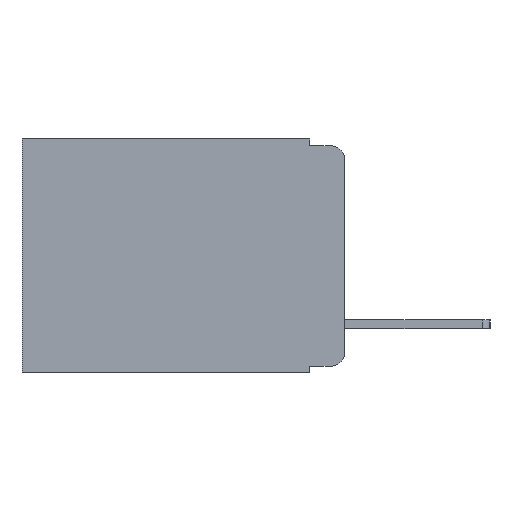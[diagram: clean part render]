
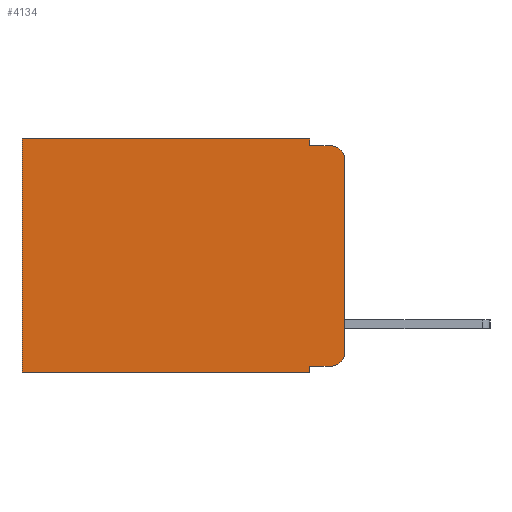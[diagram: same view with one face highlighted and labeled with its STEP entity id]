
A CAD part, left-side view. The second image highlights one B-rep face of the part: STEP entity #4134.
In plain terms, the highlighted planar face has unit normal (-1, 0, 0).
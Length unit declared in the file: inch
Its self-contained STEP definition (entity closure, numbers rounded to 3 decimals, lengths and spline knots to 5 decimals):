
#69 = LINE ( 'NONE', #575, #18979 ) ;
#92 = CARTESIAN_POINT ( 'NONE',  ( 0.298, 0.051, -0.01 ) ) ;
#381 = ORIENTED_EDGE ( 'NONE', *, *, #8845, .F. ) ;
#435 = VERTEX_POINT ( 'NONE', #7859 ) ;
#567 = DIRECTION ( 'NONE',  ( 0., 0., -1. ) ) ;
#575 = CARTESIAN_POINT ( 'NONE',  ( 0.298, 0.051, 0. ) ) ;
#897 = ORIENTED_EDGE ( 'NONE', *, *, #11427, .F. ) ;
#1057 = EDGE_CURVE ( 'NONE', #14694, #2371, #11437, .T. ) ;
#1123 = CARTESIAN_POINT ( 'NONE',  ( 0.298, 0.02, -0.03 ) ) ;
#1237 = CARTESIAN_POINT ( 'NONE',  ( 0.298, 0.051, -0.333 ) ) ;
#1401 = LINE ( 'NONE', #4087, #5179 ) ;
#1781 = LINE ( 'NONE', #4853, #9631 ) ;
#2012 = DIRECTION ( 'NONE',  ( 0., -1., 0. ) ) ;
#2315 = LINE ( 'NONE', #11335, #10576 ) ;
#2371 = VERTEX_POINT ( 'NONE', #5268 ) ;
#2662 = ORIENTED_EDGE ( 'NONE', *, *, #5626, .T. ) ;
#2708 = CARTESIAN_POINT ( 'NONE',  ( 0.298, 0., 0. ) ) ;
#3906 = LINE ( 'NONE', #92, #11995 ) ;
#4087 = CARTESIAN_POINT ( 'NONE',  ( 0.298, 0., 0. ) ) ;
#4134 = ADVANCED_FACE ( 'NONE', ( #11574 ), #5931, .F. ) ;
#4666 = ORIENTED_EDGE ( 'NONE', *, *, #1057, .T. ) ;
#4853 = CARTESIAN_POINT ( 'NONE',  ( 0.298, 0.473, 0. ) ) ;
#4934 = ORIENTED_EDGE ( 'NONE', *, *, #6023, .T. ) ;
#5108 = VERTEX_POINT ( 'NONE', #11410 ) ;
#5179 = VECTOR ( 'NONE', #17330, 39.37008 ) ;
#5268 = CARTESIAN_POINT ( 'NONE',  ( 0.298, 0.02, -0.01 ) ) ;
#5447 = DIRECTION ( 'NONE',  ( 0., 0., -1. ) ) ;
#5626 = EDGE_CURVE ( 'NONE', #11261, #17819, #2315, .T. ) ;
#5914 = VERTEX_POINT ( 'NONE', #17900 ) ;
#5924 = ORIENTED_EDGE ( 'NONE', *, *, #11070, .F. ) ;
#5931 = PLANE ( 'NONE',  #9038 ) ;
#6023 = EDGE_CURVE ( 'NONE', #15676, #435, #1781, .T. ) ;
#6117 = DIRECTION ( 'NONE',  ( -1., 0., 0. ) ) ;
#6165 = VECTOR ( 'NONE', #5447, 39.37008 ) ;
#6440 = EDGE_LOOP ( 'NONE', ( #381, #4666, #897, #9253, #10195, #4934, #17063, #5924, #2662, #8329 ) ) ;
#6445 = DIRECTION ( 'NONE',  ( 0., 0., -1. ) ) ;
#6895 = CARTESIAN_POINT ( 'NONE',  ( 0.298, 0., -0.343 ) ) ;
#7480 = DIRECTION ( 'NONE',  ( 0., 0., -1. ) ) ;
#7859 = CARTESIAN_POINT ( 'NONE',  ( 0.298, 0.473, -0.343 ) ) ;
#7922 = LINE ( 'NONE', #11811, #11399 ) ;
#8329 = ORIENTED_EDGE ( 'NONE', *, *, #8735, .T. ) ;
#8368 = CARTESIAN_POINT ( 'NONE',  ( 0.298, 0.473, 0. ) ) ;
#8735 = EDGE_CURVE ( 'NONE', #17819, #5108, #19047, .T. ) ;
#8845 = EDGE_CURVE ( 'NONE', #14694, #5108, #1401, .T. ) ;
#9038 = AXIS2_PLACEMENT_3D ( 'NONE', #2708, #16095, #7480 ) ;
#9253 = ORIENTED_EDGE ( 'NONE', *, *, #12385, .F. ) ;
#9578 = DIRECTION ( 'NONE',  ( 0., 0., -1. ) ) ;
#9631 = VECTOR ( 'NONE', #6445, 39.37008 ) ;
#9953 = DIRECTION ( 'NONE',  ( -1., 0., 0. ) ) ;
#10019 = CARTESIAN_POINT ( 'NONE',  ( 0.298, 0.051, -0.343 ) ) ;
#10064 = CARTESIAN_POINT ( 'NONE',  ( 0.298, 0.051, 0. ) ) ;
#10195 = ORIENTED_EDGE ( 'NONE', *, *, #15089, .T. ) ;
#10576 = VECTOR ( 'NONE', #2012, 39.37008 ) ;
#11009 = DIRECTION ( 'NONE',  ( 0., -1., 0. ) ) ;
#11017 = EDGE_CURVE ( 'NONE', #17611, #435, #11565, .T. ) ;
#11031 = VERTEX_POINT ( 'NONE', #11397 ) ;
#11070 = EDGE_CURVE ( 'NONE', #11261, #17611, #13983, .T. ) ;
#11099 = AXIS2_PLACEMENT_3D ( 'NONE', #1123, #6117, #9578 ) ;
#11261 = VERTEX_POINT ( 'NONE', #1237 ) ;
#11335 = CARTESIAN_POINT ( 'NONE',  ( 0.298, 0.051, -0.333 ) ) ;
#11397 = CARTESIAN_POINT ( 'NONE',  ( 0.298, 0.051, -0.01 ) ) ;
#11399 = VECTOR ( 'NONE', #14635, 39.37008 ) ;
#11410 = CARTESIAN_POINT ( 'NONE',  ( 0.298, 0., -0.313 ) ) ;
#11422 = DIRECTION ( 'NONE',  ( 0., 0., -1. ) ) ;
#11427 = EDGE_CURVE ( 'NONE', #11031, #2371, #3906, .T. ) ;
#11437 = CIRCLE ( 'NONE', #11099, 0.02 ) ;
#11565 = LINE ( 'NONE', #6895, #18593 ) ;
#11574 = FACE_OUTER_BOUND ( 'NONE', #6440, .T. ) ;
#11811 = CARTESIAN_POINT ( 'NONE',  ( 0.298, 0., 0. ) ) ;
#11995 = VECTOR ( 'NONE', #11009, 39.37008 ) ;
#12385 = EDGE_CURVE ( 'NONE', #5914, #11031, #69, .T. ) ;
#12765 = DIRECTION ( 'NONE',  ( 0., 1., 0. ) ) ;
#13366 = AXIS2_PLACEMENT_3D ( 'NONE', #18426, #9953, #567 ) ;
#13861 = CARTESIAN_POINT ( 'NONE',  ( 0.298, 0., -0.03 ) ) ;
#13983 = LINE ( 'NONE', #10064, #6165 ) ;
#14635 = DIRECTION ( 'NONE',  ( 0., 1., 0. ) ) ;
#14694 = VERTEX_POINT ( 'NONE', #13861 ) ;
#15089 = EDGE_CURVE ( 'NONE', #5914, #15676, #7922, .T. ) ;
#15676 = VERTEX_POINT ( 'NONE', #8368 ) ;
#16055 = CARTESIAN_POINT ( 'NONE',  ( 0.298, 0.02, -0.333 ) ) ;
#16095 = DIRECTION ( 'NONE',  ( 1., 0., 0. ) ) ;
#17063 = ORIENTED_EDGE ( 'NONE', *, *, #11017, .F. ) ;
#17330 = DIRECTION ( 'NONE',  ( 0., 0., -1. ) ) ;
#17611 = VERTEX_POINT ( 'NONE', #10019 ) ;
#17819 = VERTEX_POINT ( 'NONE', #16055 ) ;
#17900 = CARTESIAN_POINT ( 'NONE',  ( 0.298, 0.051, 0. ) ) ;
#18426 = CARTESIAN_POINT ( 'NONE',  ( 0.298, 0.02, -0.313 ) ) ;
#18593 = VECTOR ( 'NONE', #12765, 39.37008 ) ;
#18979 = VECTOR ( 'NONE', #11422, 39.37008 ) ;
#19047 = CIRCLE ( 'NONE', #13366, 0.02 ) ;
